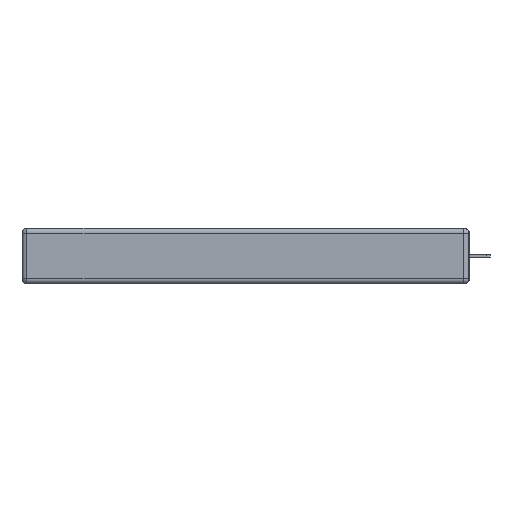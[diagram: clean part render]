
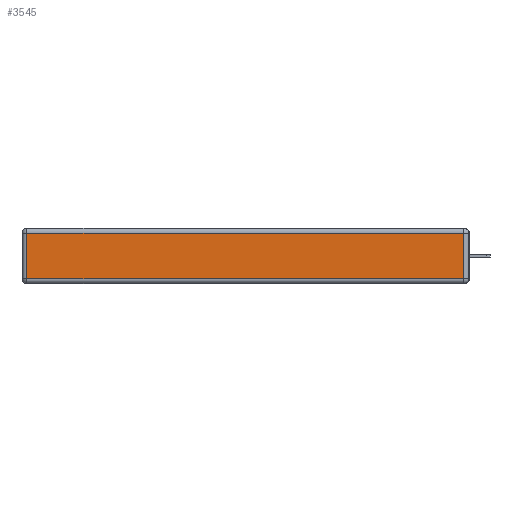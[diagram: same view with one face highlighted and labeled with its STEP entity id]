
A CAD part, left-side view. The second image highlights one B-rep face of the part: STEP entity #3545.
In plain terms, the highlighted planar face has unit normal (-1, 0, 0).
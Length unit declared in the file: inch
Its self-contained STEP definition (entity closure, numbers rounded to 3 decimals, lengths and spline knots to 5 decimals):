
#424 = VECTOR ( 'NONE', #6065, 39.37008 ) ;
#866 = PLANE ( 'NONE',  #11066 ) ;
#2116 = DIRECTION ( 'NONE',  ( 0., 0., -1. ) ) ;
#2521 = DIRECTION ( 'NONE',  ( -1., 0., 0. ) ) ;
#3545 = ADVANCED_FACE ( 'NONE', ( #14318 ), #866, .T. ) ;
#3670 = EDGE_CURVE ( 'NONE', #17423, #13843, #13214, .T. ) ;
#4881 = CARTESIAN_POINT ( 'NONE',  ( 0., 2.72, -0.343 ) ) ;
#5102 = ORIENTED_EDGE ( 'NONE', *, *, #3670, .T. ) ;
#5522 = VERTEX_POINT ( 'NONE', #18220 ) ;
#5854 = EDGE_CURVE ( 'NONE', #11678, #5522, #13379, .T. ) ;
#6037 = EDGE_CURVE ( 'NONE', #13843, #11678, #6621, .T. ) ;
#6065 = DIRECTION ( 'NONE',  ( 0., -1., 0. ) ) ;
#6250 = EDGE_LOOP ( 'NONE', ( #5102, #18011, #7094, #19115 ) ) ;
#6621 = LINE ( 'NONE', #6820, #9607 ) ;
#6820 = CARTESIAN_POINT ( 'NONE',  ( 0., 0.03, -0.343 ) ) ;
#6876 = CARTESIAN_POINT ( 'NONE',  ( 0., 0., -0.343 ) ) ;
#7094 = ORIENTED_EDGE ( 'NONE', *, *, #5854, .T. ) ;
#8788 = CARTESIAN_POINT ( 'NONE',  ( 0., 2.75, -0.03 ) ) ;
#9607 = VECTOR ( 'NONE', #17306, 39.37008 ) ;
#11066 = AXIS2_PLACEMENT_3D ( 'NONE', #6876, #2521, #13039 ) ;
#11678 = VERTEX_POINT ( 'NONE', #14575 ) ;
#13039 = DIRECTION ( 'NONE',  ( 0., 0., 1. ) ) ;
#13214 = LINE ( 'NONE', #14995, #424 ) ;
#13379 = LINE ( 'NONE', #8788, #18664 ) ;
#13843 = VERTEX_POINT ( 'NONE', #14427 ) ;
#13887 = LINE ( 'NONE', #4881, #14240 ) ;
#14240 = VECTOR ( 'NONE', #2116, 39.37008 ) ;
#14318 = FACE_OUTER_BOUND ( 'NONE', #6250, .T. ) ;
#14427 = CARTESIAN_POINT ( 'NONE',  ( 0., 0.03, -0.313 ) ) ;
#14575 = CARTESIAN_POINT ( 'NONE',  ( 0., 0.03, -0.03 ) ) ;
#14756 = DIRECTION ( 'NONE',  ( 0., 1., 0. ) ) ;
#14995 = CARTESIAN_POINT ( 'NONE',  ( 0., 0., -0.313 ) ) ;
#17033 = CARTESIAN_POINT ( 'NONE',  ( 0., 2.72, -0.313 ) ) ;
#17306 = DIRECTION ( 'NONE',  ( 0., 0., 1. ) ) ;
#17322 = EDGE_CURVE ( 'NONE', #5522, #17423, #13887, .T. ) ;
#17423 = VERTEX_POINT ( 'NONE', #17033 ) ;
#18011 = ORIENTED_EDGE ( 'NONE', *, *, #6037, .T. ) ;
#18220 = CARTESIAN_POINT ( 'NONE',  ( 0., 2.72, -0.03 ) ) ;
#18664 = VECTOR ( 'NONE', #14756, 39.37008 ) ;
#19115 = ORIENTED_EDGE ( 'NONE', *, *, #17322, .T. ) ;
